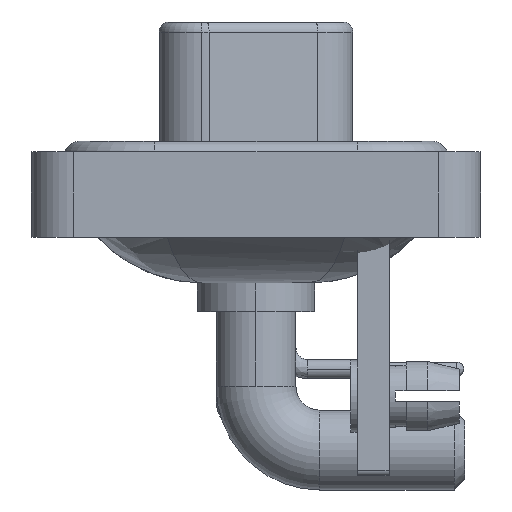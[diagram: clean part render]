
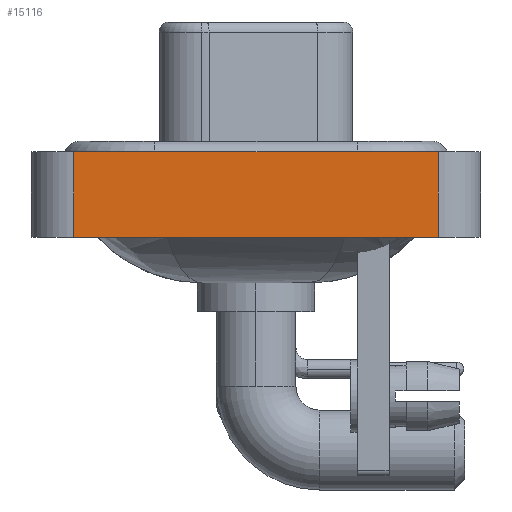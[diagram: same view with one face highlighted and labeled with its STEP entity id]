
A CAD part, left-side view. The second image highlights one B-rep face of the part: STEP entity #15116.
In plain terms, the highlighted planar face has unit normal (-1, 0, 0).
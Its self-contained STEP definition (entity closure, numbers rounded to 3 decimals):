
#595 = CARTESIAN_POINT ( 'NONE',  ( -7.35, 8.55, -3.6 ) ) ;
#2542 = PLANE ( 'NONE',  #23869 ) ;
#2706 = CARTESIAN_POINT ( 'NONE',  ( -7.35, 8.55, -3.6 ) ) ;
#3088 = VECTOR ( 'NONE', #29421, 1000. ) ;
#3542 = LINE ( 'NONE', #3704, #3088 ) ;
#3704 = CARTESIAN_POINT ( 'NONE',  ( -7.35, -8.55, -3.6 ) ) ;
#5178 = CARTESIAN_POINT ( 'NONE',  ( -7.35, -8.55, 0.4 ) ) ;
#6097 = VECTOR ( 'NONE', #26787, 1000. ) ;
#6290 = EDGE_CURVE ( 'NONE', #29186, #14002, #3542, .T. ) ;
#6897 = DIRECTION ( 'NONE',  ( 0., -1., 0. ) ) ;
#10563 = LINE ( 'NONE', #595, #6097 ) ;
#11518 = DIRECTION ( 'NONE',  ( 0., -1., 0. ) ) ;
#11912 = CARTESIAN_POINT ( 'NONE',  ( -7.35, 8.55, 0.4 ) ) ;
#12064 = EDGE_CURVE ( 'NONE', #21243, #29186, #27882, .T. ) ;
#12528 = FACE_OUTER_BOUND ( 'NONE', #27582, .T. ) ;
#14002 = VERTEX_POINT ( 'NONE', #19847 ) ;
#14267 = DIRECTION ( 'NONE',  ( 0., 0., 1. ) ) ;
#15116 = ADVANCED_FACE ( 'NONE', ( #12528 ), #2542, .T. ) ;
#17719 = ORIENTED_EDGE ( 'NONE', *, *, #12064, .T. ) ;
#17896 = VERTEX_POINT ( 'NONE', #11912 ) ;
#18831 = EDGE_CURVE ( 'NONE', #21243, #17896, #10563, .T. ) ;
#19087 = DIRECTION ( 'NONE',  ( -1., 0., 0. ) ) ;
#19847 = CARTESIAN_POINT ( 'NONE',  ( -7.35, -8.55, 0.4 ) ) ;
#20776 = VECTOR ( 'NONE', #11518, 1000. ) ;
#20789 = ORIENTED_EDGE ( 'NONE', *, *, #6290, .T. ) ;
#20924 = VECTOR ( 'NONE', #6897, 1000. ) ;
#21243 = VERTEX_POINT ( 'NONE', #2706 ) ;
#21717 = ORIENTED_EDGE ( 'NONE', *, *, #28570, .F. ) ;
#22147 = ORIENTED_EDGE ( 'NONE', *, *, #18831, .F. ) ;
#23544 = CARTESIAN_POINT ( 'NONE',  ( -7.35, -8.55, -3.6 ) ) ;
#23869 = AXIS2_PLACEMENT_3D ( 'NONE', #26272, #19087, #14267 ) ;
#25928 = LINE ( 'NONE', #5178, #20924 ) ;
#26272 = CARTESIAN_POINT ( 'NONE',  ( -7.35, -8.55, -3.6 ) ) ;
#26787 = DIRECTION ( 'NONE',  ( 0., 0., 1. ) ) ;
#27582 = EDGE_LOOP ( 'NONE', ( #20789, #21717, #22147, #17719 ) ) ;
#27858 = CARTESIAN_POINT ( 'NONE',  ( -7.35, -8.55, -3.6 ) ) ;
#27882 = LINE ( 'NONE', #23544, #20776 ) ;
#28570 = EDGE_CURVE ( 'NONE', #17896, #14002, #25928, .T. ) ;
#29186 = VERTEX_POINT ( 'NONE', #27858 ) ;
#29421 = DIRECTION ( 'NONE',  ( 0., 0., 1. ) ) ;
